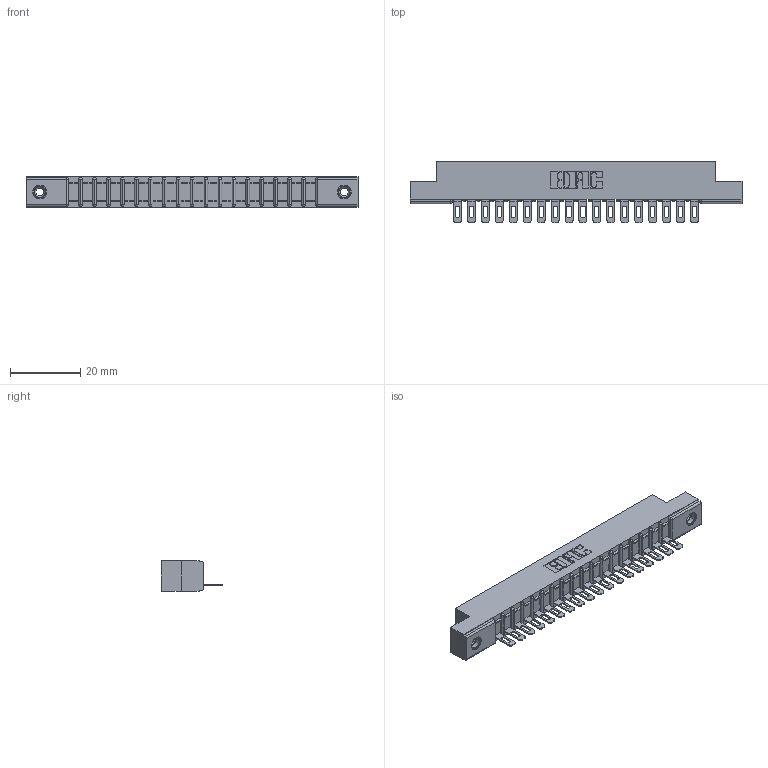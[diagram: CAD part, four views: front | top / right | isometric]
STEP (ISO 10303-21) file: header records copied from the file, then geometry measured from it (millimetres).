
FILE_DESCRIPTION (( 'STEP AP203' ), '1' );
FILE_NAME ('357-018-501-108.STEP', '2018-08-08T04:51:29', ( '' ), ( '' ), 'SwSTEP 2.0', 'SolidWorks 2016', '' );
FILE_SCHEMA (( 'CONFIG_CONTROL_DESIGN' ));
Length unit declared in the file: inch
Products named in the file (4): 357-018-501-108; 307 Part_.156 Dia Mounting Holes; 307-290-002_501; 345-250-001_345-250-003-102
Assembly tree (21 placements, depth 2):
  357-018-501-108
    307 Part_.156 Dia Mounting Holes
    307-290-002_501  x18
    345-250-001_345-250-003-102  x2
Bounding box: 94.34 x 17.42 x 8.71 mm (x, y, z)
Volume: 636 mm3; surface area: 11246.7 mm2
Topology: 20 solids, 21 shells, 1565 faces, 4743 edges, 3102 vertices
Faces by surface type: plane 894, cylinder 617, sphere 38, cone 12, torus 4
Entity records: 20369 total; most frequent: CARTESIAN_POINT 3411, ORIENTED_EDGE 3394, DIRECTION 3339, EDGE_CURVE 1697, VECTOR 1283, LINE 1283, VERTEX_POINT 1100, AXIS2_PLACEMENT_3D 1028
